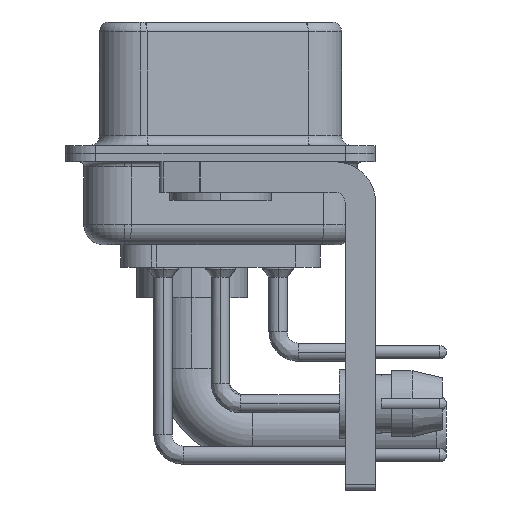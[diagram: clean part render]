
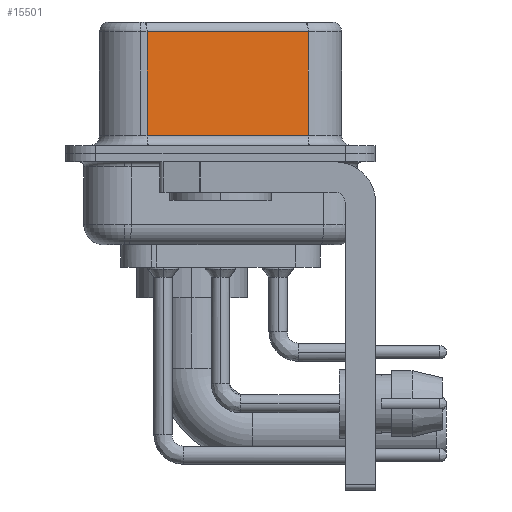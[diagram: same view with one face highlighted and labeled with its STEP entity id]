
A CAD part, left-side view. The second image highlights one B-rep face of the part: STEP entity #15501.
In plain terms, the highlighted planar face has unit normal (-0.985, -0.174, 0).
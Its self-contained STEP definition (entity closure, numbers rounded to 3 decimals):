
#964 = VECTOR ( 'NONE', #27733, 1000. ) ;
#1076 = CARTESIAN_POINT ( 'NONE',  ( 5.132, -4.322, 6.02 ) ) ;
#1320 = EDGE_CURVE ( 'NONE', #16340, #27200, #20983, .T. ) ;
#1648 = ORIENTED_EDGE ( 'NONE', *, *, #1320, .T. ) ;
#2982 = LINE ( 'NONE', #3166, #964 ) ;
#3166 = CARTESIAN_POINT ( 'NONE',  ( 5.132, -4.322, 0.9 ) ) ;
#4415 = ORIENTED_EDGE ( 'NONE', *, *, #12205, .T. ) ;
#5914 = DIRECTION ( 'NONE',  ( 0., 0., -1. ) ) ;
#10352 = EDGE_CURVE ( 'NONE', #17615, #35250, #31386, .T. ) ;
#11287 = VECTOR ( 'NONE', #39760, 1000. ) ;
#12205 = EDGE_CURVE ( 'NONE', #27200, #35250, #2982, .T. ) ;
#12531 = AXIS2_PLACEMENT_3D ( 'NONE', #23533, #20319, #20505 ) ;
#14102 = CARTESIAN_POINT ( 'NONE',  ( 3.73, 3.628, 0.9 ) ) ;
#15228 = LINE ( 'NONE', #27679, #11287 ) ;
#15501 = ADVANCED_FACE ( 'NONE', ( #23314 ), #35570, .F. ) ;
#16340 = VERTEX_POINT ( 'NONE', #31991 ) ;
#17351 = CARTESIAN_POINT ( 'NONE',  ( 3.73, 3.628, 6.52 ) ) ;
#17615 = VERTEX_POINT ( 'NONE', #1076 ) ;
#18375 = ORIENTED_EDGE ( 'NONE', *, *, #30306, .T. ) ;
#20306 = VECTOR ( 'NONE', #5914, 1000. ) ;
#20319 = DIRECTION ( 'NONE',  ( 0.985, 0.174, 0. ) ) ;
#20505 = DIRECTION ( 'NONE',  ( -0.174, 0.985, 0. ) ) ;
#20983 = LINE ( 'NONE', #17351, #37723 ) ;
#22415 = ORIENTED_EDGE ( 'NONE', *, *, #10352, .F. ) ;
#23314 = FACE_OUTER_BOUND ( 'NONE', #23663, .T. ) ;
#23533 = CARTESIAN_POINT ( 'NONE',  ( 5.132, -4.322, 6.52 ) ) ;
#23663 = EDGE_LOOP ( 'NONE', ( #22415, #18375, #1648, #4415 ) ) ;
#27200 = VERTEX_POINT ( 'NONE', #14102 ) ;
#27679 = CARTESIAN_POINT ( 'NONE',  ( 5.132, -4.322, 6.02 ) ) ;
#27733 = DIRECTION ( 'NONE',  ( 0.174, -0.985, 0. ) ) ;
#30306 = EDGE_CURVE ( 'NONE', #17615, #16340, #15228, .T. ) ;
#31386 = LINE ( 'NONE', #31783, #20306 ) ;
#31783 = CARTESIAN_POINT ( 'NONE',  ( 5.132, -4.322, 6.52 ) ) ;
#31991 = CARTESIAN_POINT ( 'NONE',  ( 3.73, 3.628, 6.02 ) ) ;
#35250 = VERTEX_POINT ( 'NONE', #36503 ) ;
#35570 = PLANE ( 'NONE',  #12531 ) ;
#36446 = DIRECTION ( 'NONE',  ( 0., 0., -1. ) ) ;
#36503 = CARTESIAN_POINT ( 'NONE',  ( 5.132, -4.322, 0.9 ) ) ;
#37723 = VECTOR ( 'NONE', #36446, 1000. ) ;
#39760 = DIRECTION ( 'NONE',  ( -0.174, 0.985, 0. ) ) ;
